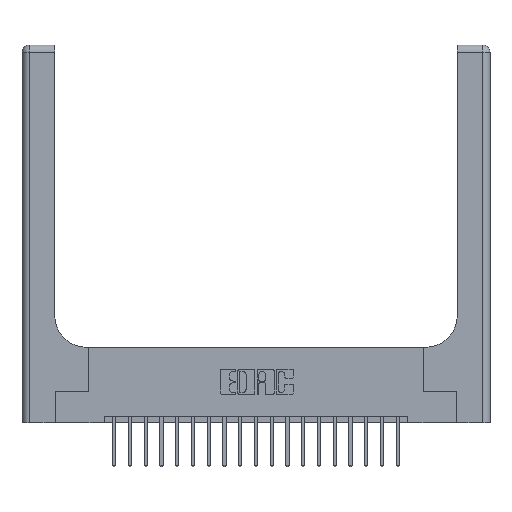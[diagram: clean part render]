
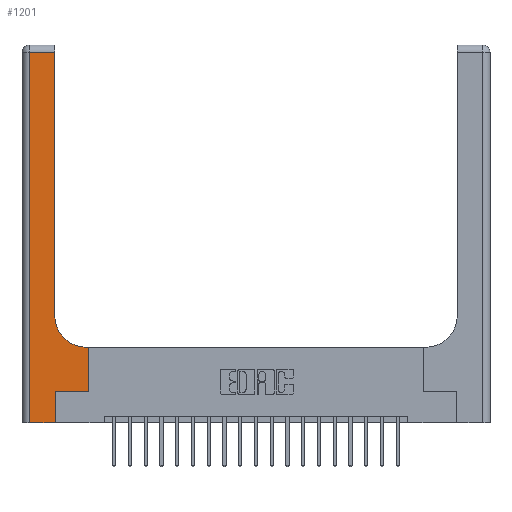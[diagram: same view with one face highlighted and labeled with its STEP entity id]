
A CAD part, top view. The second image highlights one B-rep face of the part: STEP entity #1201.
In plain terms, the highlighted planar face has unit normal (0, 0, 1).
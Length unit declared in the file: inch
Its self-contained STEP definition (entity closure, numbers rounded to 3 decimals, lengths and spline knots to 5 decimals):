
#550 = CARTESIAN_POINT ( 'NONE',  ( 0.06, 2.94, 0.37 ) ) ;
#853 = DIRECTION ( 'NONE',  ( 1., 0., 0. ) ) ;
#974 = CARTESIAN_POINT ( 'NONE',  ( 0.26, 0.85, 0.37 ) ) ;
#1201 = ADVANCED_FACE ( 'NONE', ( #4624 ), #19678, .F. ) ;
#1415 = DIRECTION ( 'NONE',  ( -1., 0., 0. ) ) ;
#1658 = LINE ( 'NONE', #8060, #12286 ) ;
#1695 = CARTESIAN_POINT ( 'NONE',  ( 0.265, 0., 0.37 ) ) ;
#1715 = VERTEX_POINT ( 'NONE', #5230 ) ;
#1931 = ORIENTED_EDGE ( 'NONE', *, *, #11477, .T. ) ;
#2181 = LINE ( 'NONE', #3690, #20476 ) ;
#2415 = ORIENTED_EDGE ( 'NONE', *, *, #2955, .T. ) ;
#2562 = LINE ( 'NONE', #10570, #20024 ) ;
#2916 = EDGE_CURVE ( 'NONE', #18601, #19899, #14267, .T. ) ;
#2953 = DIRECTION ( 'NONE',  ( 0., -1., 0. ) ) ;
#2955 = EDGE_CURVE ( 'NONE', #15364, #6372, #6631, .T. ) ;
#3071 = CARTESIAN_POINT ( 'NONE',  ( 0.265, 0., 0.37 ) ) ;
#3136 = EDGE_LOOP ( 'NONE', ( #6217, #2415, #1931, #10968, #13696, #6429, #11324, #11936, #12371 ) ) ;
#3690 = CARTESIAN_POINT ( 'NONE',  ( 0.26, 0.6, 0.37 ) ) ;
#4624 = FACE_OUTER_BOUND ( 'NONE', #3136, .T. ) ;
#5033 = DIRECTION ( 'NONE',  ( -1., 0., 0. ) ) ;
#5111 = EDGE_CURVE ( 'NONE', #1715, #19690, #20150, .T. ) ;
#5230 = CARTESIAN_POINT ( 'NONE',  ( 0.265, 0.25, 0.37 ) ) ;
#5585 = VECTOR ( 'NONE', #16432, 39.37008 ) ;
#5625 = CARTESIAN_POINT ( 'NONE',  ( 0.265, 0.25, 0.37 ) ) ;
#6217 = ORIENTED_EDGE ( 'NONE', *, *, #15729, .T. ) ;
#6372 = VERTEX_POINT ( 'NONE', #550 ) ;
#6429 = ORIENTED_EDGE ( 'NONE', *, *, #5111, .T. ) ;
#6523 = DIRECTION ( 'NONE',  ( 0., 0., -1. ) ) ;
#6631 = LINE ( 'NONE', #10130, #7428 ) ;
#6734 = CARTESIAN_POINT ( 'NONE',  ( 0.51, 0.85, 0.37 ) ) ;
#6897 = CARTESIAN_POINT ( 'NONE',  ( 0.26, 3., 0.37 ) ) ;
#7103 = CARTESIAN_POINT ( 'NONE',  ( 0.51, 0.6, 0.37 ) ) ;
#7420 = DIRECTION ( 'NONE',  ( 1., 0., 0. ) ) ;
#7428 = VECTOR ( 'NONE', #5033, 39.37008 ) ;
#8019 = DIRECTION ( 'NONE',  ( 0., 0., -1. ) ) ;
#8028 = EDGE_CURVE ( 'NONE', #19690, #9744, #16643, .T. ) ;
#8060 = CARTESIAN_POINT ( 'NONE',  ( 0.06, 3., 0.37 ) ) ;
#8183 = VECTOR ( 'NONE', #16137, 39.37008 ) ;
#8701 = LINE ( 'NONE', #6897, #17049 ) ;
#8933 = VERTEX_POINT ( 'NONE', #18289 ) ;
#9052 = EDGE_CURVE ( 'NONE', #12943, #1715, #9599, .T. ) ;
#9599 = LINE ( 'NONE', #1695, #8183 ) ;
#9744 = VERTEX_POINT ( 'NONE', #13844 ) ;
#9904 = CARTESIAN_POINT ( 'NONE',  ( 0.528, 0.25, 0.37 ) ) ;
#10130 = CARTESIAN_POINT ( 'NONE',  ( 0., 2.94, 0.37 ) ) ;
#10246 = EDGE_CURVE ( 'NONE', #8933, #12943, #2562, .T. ) ;
#10570 = CARTESIAN_POINT ( 'NONE',  ( 0., 0., 0.37 ) ) ;
#10968 = ORIENTED_EDGE ( 'NONE', *, *, #10246, .T. ) ;
#11324 = ORIENTED_EDGE ( 'NONE', *, *, #8028, .T. ) ;
#11332 = CARTESIAN_POINT ( 'NONE',  ( 0.26, 2.94, 0.37 ) ) ;
#11477 = EDGE_CURVE ( 'NONE', #6372, #8933, #1658, .T. ) ;
#11936 = ORIENTED_EDGE ( 'NONE', *, *, #15681, .T. ) ;
#12286 = VECTOR ( 'NONE', #2953, 39.37008 ) ;
#12371 = ORIENTED_EDGE ( 'NONE', *, *, #2916, .T. ) ;
#12943 = VERTEX_POINT ( 'NONE', #3071 ) ;
#13046 = DIRECTION ( 'NONE',  ( 1., 0., 0. ) ) ;
#13606 = VECTOR ( 'NONE', #7420, 39.37008 ) ;
#13696 = ORIENTED_EDGE ( 'NONE', *, *, #9052, .T. ) ;
#13844 = CARTESIAN_POINT ( 'NONE',  ( 0.528, 0.6, 0.37 ) ) ;
#14267 = CIRCLE ( 'NONE', #17679, 0.25 ) ;
#14762 = CARTESIAN_POINT ( 'NONE',  ( 0., 3., 0.37 ) ) ;
#15245 = DIRECTION ( 'NONE',  ( 0., 1., 0. ) ) ;
#15364 = VERTEX_POINT ( 'NONE', #11332 ) ;
#15681 = EDGE_CURVE ( 'NONE', #9744, #18601, #2181, .T. ) ;
#15729 = EDGE_CURVE ( 'NONE', #19899, #15364, #8701, .T. ) ;
#16137 = DIRECTION ( 'NONE',  ( 0., 1., 0. ) ) ;
#16212 = AXIS2_PLACEMENT_3D ( 'NONE', #14762, #8019, #1415 ) ;
#16432 = DIRECTION ( 'NONE',  ( 0., 1., 0. ) ) ;
#16522 = DIRECTION ( 'NONE',  ( -1., 0., 0. ) ) ;
#16643 = LINE ( 'NONE', #9904, #5585 ) ;
#17049 = VECTOR ( 'NONE', #15245, 39.37008 ) ;
#17679 = AXIS2_PLACEMENT_3D ( 'NONE', #6734, #6523, #13046 ) ;
#18289 = CARTESIAN_POINT ( 'NONE',  ( 0.06, 0., 0.37 ) ) ;
#18371 = CARTESIAN_POINT ( 'NONE',  ( 0.528, 0.25, 0.37 ) ) ;
#18601 = VERTEX_POINT ( 'NONE', #7103 ) ;
#19678 = PLANE ( 'NONE',  #16212 ) ;
#19690 = VERTEX_POINT ( 'NONE', #18371 ) ;
#19899 = VERTEX_POINT ( 'NONE', #974 ) ;
#20024 = VECTOR ( 'NONE', #853, 39.37008 ) ;
#20150 = LINE ( 'NONE', #5625, #13606 ) ;
#20476 = VECTOR ( 'NONE', #16522, 39.37008 ) ;
